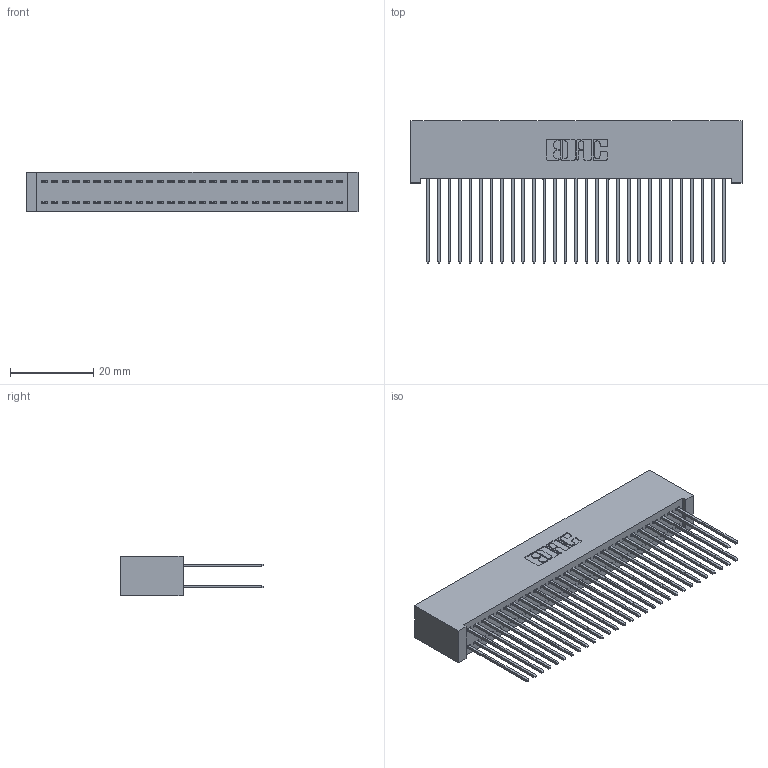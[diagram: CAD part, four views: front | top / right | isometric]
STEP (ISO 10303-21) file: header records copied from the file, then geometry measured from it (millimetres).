
FILE_DESCRIPTION (( 'STEP AP203' ), '1' );
FILE_NAME ('342-058-541-201.STEP', '2019-10-03T12:45:48', ( '' ), ( '' ), 'SwSTEP 2.0', 'SolidWorks 2016', '' );
FILE_SCHEMA (( 'CONFIG_CONTROL_DESIGN' ));
Length unit declared in the file: inch
Products named in the file (3): 342-058-541-201; 342 Part_Lugless; 345-292-001_345-293-141
Assembly tree (59 placements, depth 2):
  342-058-541-201
    342 Part_Lugless
    345-292-001_345-293-141  x58
Bounding box: 79.91 x 34.3 x 9.4 mm (x, y, z)
Volume: 7890.5 mm3; surface area: 14474.3 mm2
Topology: 59 solids, 59 shells, 3118 faces, 9265 edges, 6098 vertices
Faces by surface type: plane 2150, cylinder 968
Entity records: 19947 total; most frequent: CARTESIAN_POINT 3318, ORIENTED_EDGE 3254, DIRECTION 2851, EDGE_CURVE 1627, LINE 1507, VECTOR 1507, VERTEX_POINT 1082, AXIS2_PLACEMENT_3D 672
